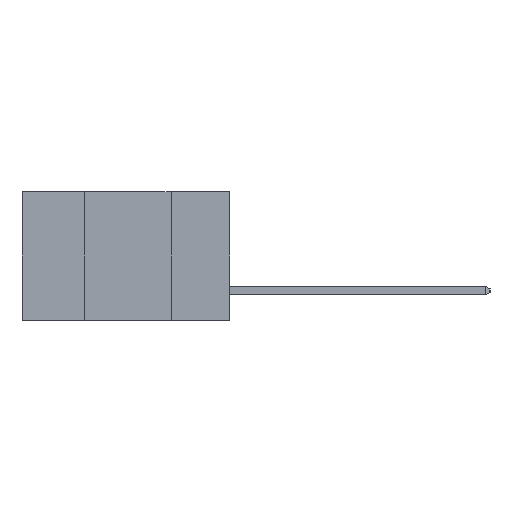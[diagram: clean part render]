
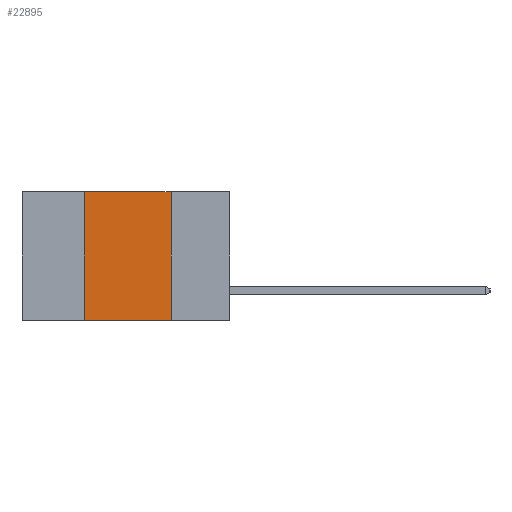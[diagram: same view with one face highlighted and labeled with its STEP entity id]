
A CAD part, left-side view. The second image highlights one B-rep face of the part: STEP entity #22895.
In plain terms, the highlighted planar face has unit normal (-1, 0, 0).
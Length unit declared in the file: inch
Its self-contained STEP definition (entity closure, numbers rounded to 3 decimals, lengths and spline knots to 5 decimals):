
#119 = DIRECTION ( 'NONE',  ( 0., 0., 1. ) ) ;
#356 = LINE ( 'NONE', #13531, #10377 ) ;
#1858 = CARTESIAN_POINT ( 'NONE',  ( 0., 0.42, -0.37 ) ) ;
#2329 = LINE ( 'NONE', #22901, #23943 ) ;
#6753 = EDGE_CURVE ( 'NONE', #21234, #25516, #8392, .T. ) ;
#7778 = CARTESIAN_POINT ( 'NONE',  ( 0., 0.17, 0. ) ) ;
#8392 = LINE ( 'NONE', #17597, #13996 ) ;
#10377 = VECTOR ( 'NONE', #17740, 39.37008 ) ;
#11216 = FACE_OUTER_BOUND ( 'NONE', #13952, .T. ) ;
#12130 = CARTESIAN_POINT ( 'NONE',  ( 0., 0.6, 0. ) ) ;
#12594 = DIRECTION ( 'NONE',  ( 0., 0., -1. ) ) ;
#12732 = ORIENTED_EDGE ( 'NONE', *, *, #24420, .F. ) ;
#12838 = CARTESIAN_POINT ( 'NONE',  ( 0., 0.42, 0. ) ) ;
#13050 = EDGE_CURVE ( 'NONE', #25491, #25516, #2329, .T. ) ;
#13531 = CARTESIAN_POINT ( 'NONE',  ( 0., 0.6, 0. ) ) ;
#13952 = EDGE_LOOP ( 'NONE', ( #23091, #25948, #12732, #17611 ) ) ;
#13996 = VECTOR ( 'NONE', #19662, 39.37008 ) ;
#14155 = CARTESIAN_POINT ( 'NONE',  ( 0., 0.17, -0.37 ) ) ;
#14223 = DIRECTION ( 'NONE',  ( 0., 0., -1. ) ) ;
#15910 = VERTEX_POINT ( 'NONE', #16539 ) ;
#16237 = PLANE ( 'NONE',  #17518 ) ;
#16539 = CARTESIAN_POINT ( 'NONE',  ( 0., 0.42, 0. ) ) ;
#17518 = AXIS2_PLACEMENT_3D ( 'NONE', #12130, #26564, #14223 ) ;
#17597 = CARTESIAN_POINT ( 'NONE',  ( 0., 0.6, -0.37 ) ) ;
#17611 = ORIENTED_EDGE ( 'NONE', *, *, #6753, .T. ) ;
#17740 = DIRECTION ( 'NONE',  ( 0., -1., 0. ) ) ;
#19605 = VECTOR ( 'NONE', #119, 39.37008 ) ;
#19662 = DIRECTION ( 'NONE',  ( 0., -1., 0. ) ) ;
#20252 = LINE ( 'NONE', #12838, #19605 ) ;
#21234 = VERTEX_POINT ( 'NONE', #1858 ) ;
#22895 = ADVANCED_FACE ( 'NONE', ( #11216 ), #16237, .F. ) ;
#22901 = CARTESIAN_POINT ( 'NONE',  ( 0., 0.17, 0. ) ) ;
#23091 = ORIENTED_EDGE ( 'NONE', *, *, #13050, .F. ) ;
#23943 = VECTOR ( 'NONE', #12594, 39.37008 ) ;
#24420 = EDGE_CURVE ( 'NONE', #21234, #15910, #20252, .T. ) ;
#25491 = VERTEX_POINT ( 'NONE', #7778 ) ;
#25516 = VERTEX_POINT ( 'NONE', #14155 ) ;
#25948 = ORIENTED_EDGE ( 'NONE', *, *, #26389, .F. ) ;
#26389 = EDGE_CURVE ( 'NONE', #15910, #25491, #356, .T. ) ;
#26564 = DIRECTION ( 'NONE',  ( 1., 0., 0. ) ) ;
